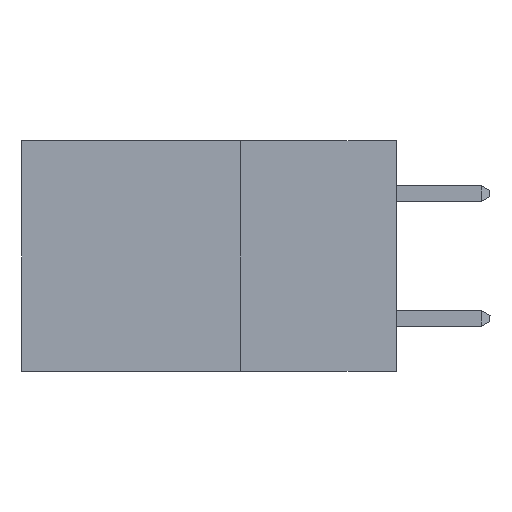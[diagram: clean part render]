
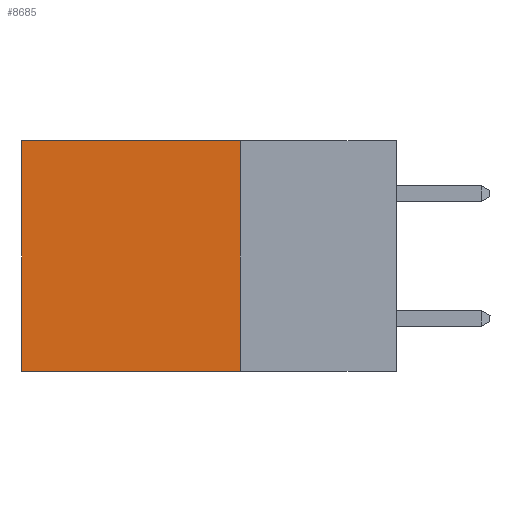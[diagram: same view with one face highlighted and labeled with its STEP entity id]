
A CAD part, left-side view. The second image highlights one B-rep face of the part: STEP entity #8685.
In plain terms, the highlighted planar face has unit normal (-1, 0, 0).
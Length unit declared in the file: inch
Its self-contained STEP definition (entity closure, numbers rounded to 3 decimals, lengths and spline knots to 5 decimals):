
#831 = PLANE ( 'NONE',  #19995 ) ;
#1234 = EDGE_CURVE ( 'NONE', #4154, #12330, #7857, .T. ) ;
#1432 = EDGE_CURVE ( 'NONE', #6576, #4154, #17455, .T. ) ;
#2937 = ORIENTED_EDGE ( 'NONE', *, *, #1234, .T. ) ;
#3660 = CARTESIAN_POINT ( 'NONE',  ( 0.2615, 0.6, 0. ) ) ;
#4154 = VERTEX_POINT ( 'NONE', #3660 ) ;
#4758 = EDGE_CURVE ( 'NONE', #6576, #14020, #17858, .T. ) ;
#4960 = DIRECTION ( 'NONE',  ( 0., 1., 0. ) ) ;
#5463 = LINE ( 'NONE', #15517, #10186 ) ;
#6338 = CARTESIAN_POINT ( 'NONE',  ( 0.2615, 0.25, 0. ) ) ;
#6576 = VERTEX_POINT ( 'NONE', #6338 ) ;
#7025 = CARTESIAN_POINT ( 'NONE',  ( 0.2615, 0.25, -0.37 ) ) ;
#7303 = VECTOR ( 'NONE', #13472, 39.37008 ) ;
#7857 = LINE ( 'NONE', #13929, #7303 ) ;
#8033 = CARTESIAN_POINT ( 'NONE',  ( 0.2615, 0.25, 0. ) ) ;
#8199 = DIRECTION ( 'NONE',  ( 0., 1., 0. ) ) ;
#8685 = ADVANCED_FACE ( 'NONE', ( #19613 ), #831, .F. ) ;
#9672 = DIRECTION ( 'NONE',  ( 1., 0., 0. ) ) ;
#10084 = ORIENTED_EDGE ( 'NONE', *, *, #1432, .T. ) ;
#10186 = VECTOR ( 'NONE', #4960, 39.37008 ) ;
#10670 = DIRECTION ( 'NONE',  ( 0., 0., -1. ) ) ;
#12228 = ORIENTED_EDGE ( 'NONE', *, *, #17812, .F. ) ;
#12257 = VECTOR ( 'NONE', #8199, 39.37008 ) ;
#12330 = VERTEX_POINT ( 'NONE', #17249 ) ;
#13235 = VECTOR ( 'NONE', #10670, 39.37008 ) ;
#13472 = DIRECTION ( 'NONE',  ( 0., 0., -1. ) ) ;
#13929 = CARTESIAN_POINT ( 'NONE',  ( 0.2615, 0.6, -0.37 ) ) ;
#14020 = VERTEX_POINT ( 'NONE', #7025 ) ;
#14765 = ORIENTED_EDGE ( 'NONE', *, *, #4758, .F. ) ;
#15449 = EDGE_LOOP ( 'NONE', ( #2937, #12228, #14765, #10084 ) ) ;
#15517 = CARTESIAN_POINT ( 'NONE',  ( 0.2615, 0.25, -0.37 ) ) ;
#15795 = CARTESIAN_POINT ( 'NONE',  ( 0.2615, 0.25, -0.37 ) ) ;
#17249 = CARTESIAN_POINT ( 'NONE',  ( 0.2615, 0.6, -0.37 ) ) ;
#17455 = LINE ( 'NONE', #8033, #12257 ) ;
#17812 = EDGE_CURVE ( 'NONE', #14020, #12330, #5463, .T. ) ;
#17858 = LINE ( 'NONE', #15795, #13235 ) ;
#18366 = CARTESIAN_POINT ( 'NONE',  ( 0.2615, 0.25, -0.37 ) ) ;
#19613 = FACE_OUTER_BOUND ( 'NONE', #15449, .T. ) ;
#19995 = AXIS2_PLACEMENT_3D ( 'NONE', #18366, #9672, #21815 ) ;
#21815 = DIRECTION ( 'NONE',  ( 0., 0., -1. ) ) ;
